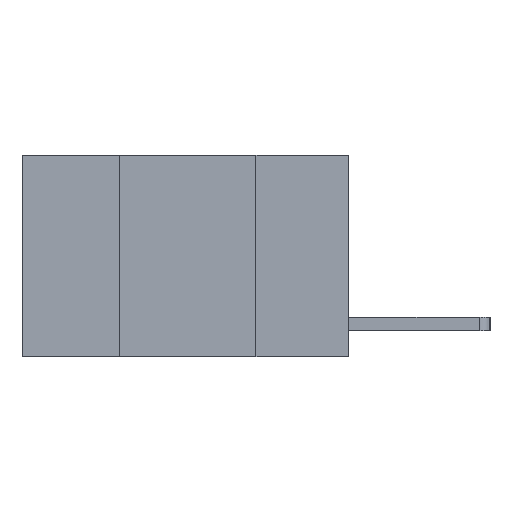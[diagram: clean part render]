
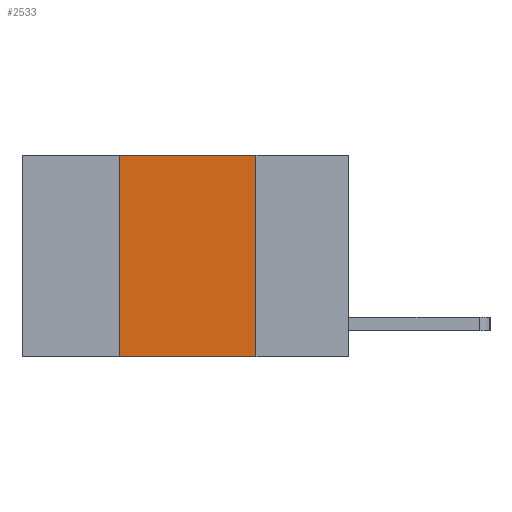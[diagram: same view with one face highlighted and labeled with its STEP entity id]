
A CAD part, left-side view. The second image highlights one B-rep face of the part: STEP entity #2533.
In plain terms, the highlighted planar face has unit normal (-1, 0, 0).
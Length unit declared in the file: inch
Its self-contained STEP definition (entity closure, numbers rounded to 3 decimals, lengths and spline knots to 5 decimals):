
#398 = EDGE_CURVE ( 'NONE', #8594, #3447, #559, .T. ) ;
#433 = CARTESIAN_POINT ( 'NONE',  ( 0., 0.42, -0.37 ) ) ;
#559 = LINE ( 'NONE', #7082, #7396 ) ;
#696 = VECTOR ( 'NONE', #3761, 39.37008 ) ;
#786 = VERTEX_POINT ( 'NONE', #3528 ) ;
#1328 = EDGE_LOOP ( 'NONE', ( #4496, #5918, #4599, #8287 ) ) ;
#1865 = CARTESIAN_POINT ( 'NONE',  ( 0., 0.17, 0. ) ) ;
#2533 = ADVANCED_FACE ( 'NONE', ( #3168 ), #3703, .F. ) ;
#2621 = DIRECTION ( 'NONE',  ( 0., -1., 0. ) ) ;
#2628 = CARTESIAN_POINT ( 'NONE',  ( 0., 0.17, 0. ) ) ;
#2728 = CARTESIAN_POINT ( 'NONE',  ( 0., 0.17, -0.37 ) ) ;
#2806 = EDGE_CURVE ( 'NONE', #4542, #3447, #5034, .T. ) ;
#3168 = FACE_OUTER_BOUND ( 'NONE', #1328, .T. ) ;
#3447 = VERTEX_POINT ( 'NONE', #2728 ) ;
#3528 = CARTESIAN_POINT ( 'NONE',  ( 0., 0.42, 0. ) ) ;
#3703 = PLANE ( 'NONE',  #8527 ) ;
#3761 = DIRECTION ( 'NONE',  ( 0., -1., 0. ) ) ;
#4362 = DIRECTION ( 'NONE',  ( 0., 0., -1. ) ) ;
#4424 = CARTESIAN_POINT ( 'NONE',  ( 0., 0.6, 0. ) ) ;
#4440 = EDGE_CURVE ( 'NONE', #786, #4542, #6013, .T. ) ;
#4496 = ORIENTED_EDGE ( 'NONE', *, *, #2806, .F. ) ;
#4542 = VERTEX_POINT ( 'NONE', #1865 ) ;
#4599 = ORIENTED_EDGE ( 'NONE', *, *, #6381, .F. ) ;
#4870 = CARTESIAN_POINT ( 'NONE',  ( 0., 0.42, 0. ) ) ;
#5034 = LINE ( 'NONE', #2628, #6345 ) ;
#5383 = LINE ( 'NONE', #4870, #6923 ) ;
#5628 = CARTESIAN_POINT ( 'NONE',  ( 0., 0.6, 0. ) ) ;
#5918 = ORIENTED_EDGE ( 'NONE', *, *, #4440, .F. ) ;
#6013 = LINE ( 'NONE', #4424, #696 ) ;
#6345 = VECTOR ( 'NONE', #7209, 39.37008 ) ;
#6381 = EDGE_CURVE ( 'NONE', #8594, #786, #5383, .T. ) ;
#6810 = DIRECTION ( 'NONE',  ( 0., 0., 1. ) ) ;
#6923 = VECTOR ( 'NONE', #6810, 39.37008 ) ;
#7082 = CARTESIAN_POINT ( 'NONE',  ( 0., 0.6, -0.37 ) ) ;
#7209 = DIRECTION ( 'NONE',  ( 0., 0., -1. ) ) ;
#7396 = VECTOR ( 'NONE', #2621, 39.37008 ) ;
#8287 = ORIENTED_EDGE ( 'NONE', *, *, #398, .T. ) ;
#8288 = DIRECTION ( 'NONE',  ( 1., 0., 0. ) ) ;
#8527 = AXIS2_PLACEMENT_3D ( 'NONE', #5628, #8288, #4362 ) ;
#8594 = VERTEX_POINT ( 'NONE', #433 ) ;
